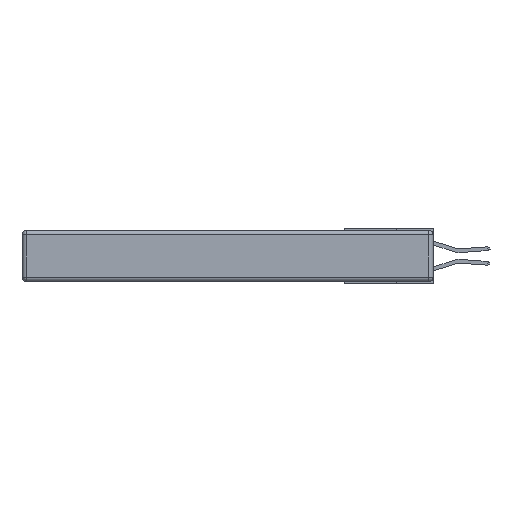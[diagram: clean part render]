
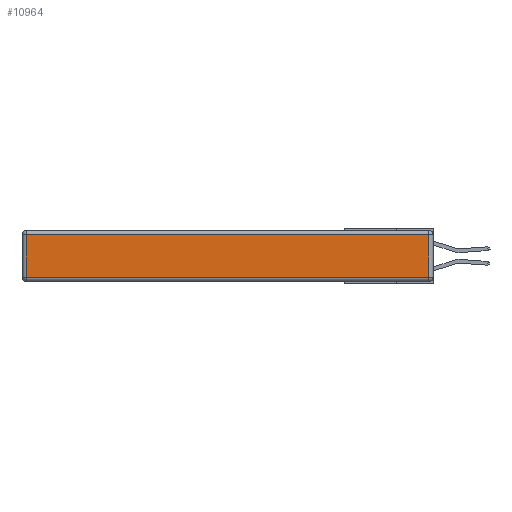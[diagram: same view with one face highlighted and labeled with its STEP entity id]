
A CAD part, left-side view. The second image highlights one B-rep face of the part: STEP entity #10964.
In plain terms, the highlighted planar face has unit normal (-1, 0, 0).
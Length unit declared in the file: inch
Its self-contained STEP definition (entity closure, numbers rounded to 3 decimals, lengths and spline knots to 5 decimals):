
#209 = ORIENTED_EDGE ( 'NONE', *, *, #5775, .T. ) ;
#557 = ORIENTED_EDGE ( 'NONE', *, *, #11391, .T. ) ;
#3001 = CARTESIAN_POINT ( 'NONE',  ( 0., 0.03, -0.343 ) ) ;
#3086 = DIRECTION ( 'NONE',  ( 0., 0., 1. ) ) ;
#3137 = VERTEX_POINT ( 'NONE', #17837 ) ;
#3769 = VERTEX_POINT ( 'NONE', #12473 ) ;
#3789 = AXIS2_PLACEMENT_3D ( 'NONE', #23527, #4857, #14248 ) ;
#4396 = VECTOR ( 'NONE', #14195, 39.37008 ) ;
#4577 = LINE ( 'NONE', #3001, #12043 ) ;
#4857 = DIRECTION ( 'NONE',  ( -1., 0., 0. ) ) ;
#5775 = EDGE_CURVE ( 'NONE', #17832, #3137, #8764, .T. ) ;
#5824 = VECTOR ( 'NONE', #18788, 39.37008 ) ;
#8764 = LINE ( 'NONE', #20661, #9609 ) ;
#9609 = VECTOR ( 'NONE', #16805, 39.37008 ) ;
#10687 = LINE ( 'NONE', #22564, #5824 ) ;
#10964 = ADVANCED_FACE ( 'NONE', ( #15804 ), #18025, .T. ) ;
#11076 = EDGE_LOOP ( 'NONE', ( #16375, #557, #209, #22497 ) ) ;
#11170 = VERTEX_POINT ( 'NONE', #20692 ) ;
#11391 = EDGE_CURVE ( 'NONE', #11170, #17832, #4577, .T. ) ;
#12043 = VECTOR ( 'NONE', #3086, 39.37008 ) ;
#12473 = CARTESIAN_POINT ( 'NONE',  ( 0., 2.72, -0.313 ) ) ;
#14195 = DIRECTION ( 'NONE',  ( 0., 0., -1. ) ) ;
#14248 = DIRECTION ( 'NONE',  ( 0., 0., 1. ) ) ;
#15025 = LINE ( 'NONE', #21566, #4396 ) ;
#15804 = FACE_OUTER_BOUND ( 'NONE', #11076, .T. ) ;
#16375 = ORIENTED_EDGE ( 'NONE', *, *, #18807, .T. ) ;
#16805 = DIRECTION ( 'NONE',  ( 0., 1., 0. ) ) ;
#17394 = CARTESIAN_POINT ( 'NONE',  ( 0., 0.03, -0.03 ) ) ;
#17832 = VERTEX_POINT ( 'NONE', #17394 ) ;
#17837 = CARTESIAN_POINT ( 'NONE',  ( 0., 2.72, -0.03 ) ) ;
#18025 = PLANE ( 'NONE',  #3789 ) ;
#18646 = EDGE_CURVE ( 'NONE', #3137, #3769, #15025, .T. ) ;
#18788 = DIRECTION ( 'NONE',  ( 0., -1., 0. ) ) ;
#18807 = EDGE_CURVE ( 'NONE', #3769, #11170, #10687, .T. ) ;
#20661 = CARTESIAN_POINT ( 'NONE',  ( 0., 2.75, -0.03 ) ) ;
#20692 = CARTESIAN_POINT ( 'NONE',  ( 0., 0.03, -0.313 ) ) ;
#21566 = CARTESIAN_POINT ( 'NONE',  ( 0., 2.72, -0.343 ) ) ;
#22497 = ORIENTED_EDGE ( 'NONE', *, *, #18646, .T. ) ;
#22564 = CARTESIAN_POINT ( 'NONE',  ( 0., 0., -0.313 ) ) ;
#23527 = CARTESIAN_POINT ( 'NONE',  ( 0., 0., -0.343 ) ) ;
